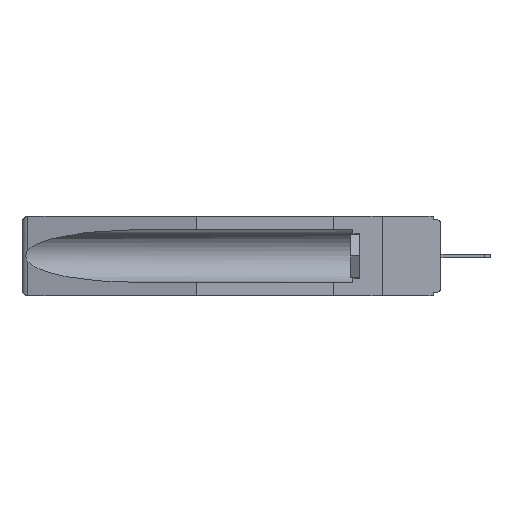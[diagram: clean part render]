
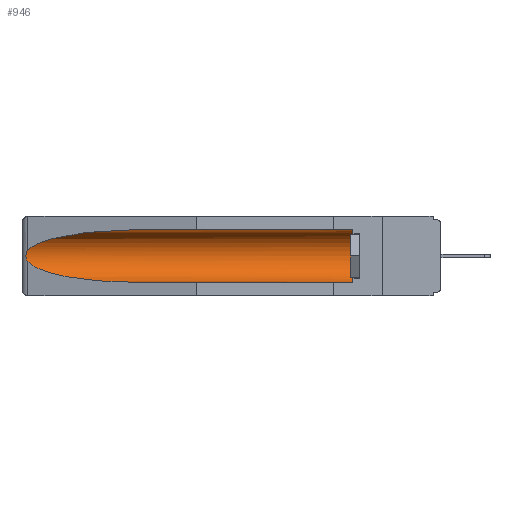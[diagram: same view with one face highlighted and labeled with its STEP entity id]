
A CAD part, left-side view. The second image highlights one B-rep face of the part: STEP entity #946.
In plain terms, the highlighted cylindrical face has radius 2.857 mm (diameter 5.715 mm), a partial arc.
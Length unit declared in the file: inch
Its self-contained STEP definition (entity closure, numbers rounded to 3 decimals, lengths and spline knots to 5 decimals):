
#84 = B_SPLINE_CURVE_WITH_KNOTS ( 'NONE', 3,
 ( #17171, #11885, #2323, #2411, #3823, #6759, #2582, #14613, #9230, #10562 ),
 .UNSPECIFIED., .F., .F.,
 ( 4, 2, 2, 2, 4 ),
 ( 0., 0.00029, 0.00058, 0.00087, 0.00117 ),
 .UNSPECIFIED. ) ;
#172 = VERTEX_POINT ( 'NONE', #4452 ) ;
#292 = CARTESIAN_POINT ( 'NONE',  ( 0.155, 0.126, -0.1715 ) ) ;
#384 = DIRECTION ( 'NONE',  ( 0., -1., 0. ) ) ;
#946 = ADVANCED_FACE ( 'NONE', ( #11473 ), #6060, .F. ) ;
#1336 = CARTESIAN_POINT ( 'NONE',  ( 0.155, -0.30754, -0.284 ) ) ;
#1440 = VECTOR ( 'NONE', #9581, 39.37008 ) ;
#1489 = CARTESIAN_POINT ( 'NONE',  ( 0.155, 1.07973, -0.284 ) ) ;
#1617 = CARTESIAN_POINT ( 'NONE',  ( 0.155, 0.126, -0.284 ) ) ;
#1957 = ORIENTED_EDGE ( 'NONE', *, *, #6160, .F. ) ;
#2323 = CARTESIAN_POINT ( 'NONE',  ( 0.26654, 1.53092, -0.15636 ) ) ;
#2411 = CARTESIAN_POINT ( 'NONE',  ( 0.2673, 1.5327, -0.16383 ) ) ;
#2578 = VECTOR ( 'NONE', #17317, 39.37008 ) ;
#2582 = CARTESIAN_POINT ( 'NONE',  ( 0.2673, 1.53269, -0.17917 ) ) ;
#2665 = ORIENTED_EDGE ( 'NONE', *, *, #8101, .T. ) ;
#2955 = AXIS2_PLACEMENT_3D ( 'NONE', #292, #384, #9781 ) ;
#3110 = CARTESIAN_POINT ( 'NONE',  ( 0.155, 0.126, -0.059 ) ) ;
#3131 = CARTESIAN_POINT ( 'NONE',  ( 0.21114, 1.30732, -0.284 ) ) ;
#3823 = CARTESIAN_POINT ( 'NONE',  ( 0.2675, 1.53308, -0.16763 ) ) ;
#4207 = CARTESIAN_POINT ( 'NONE',  ( 0.155, 1.07973, -0.284 ) ) ;
#4452 = CARTESIAN_POINT ( 'NONE',  ( 0.26537, 1.52718, -0.14972 ) ) ;
#4472 = CARTESIAN_POINT ( 'NONE',  ( 0.26537, 1.52718, -0.19328 ) ) ;
#4498 = ORIENTED_EDGE ( 'NONE', *, *, #11284, .T. ) ;
#4555 = CARTESIAN_POINT ( 'NONE',  ( 0.155, -0.30754, -0.1715 ) ) ;
#5456 = CARTESIAN_POINT ( 'NONE',  ( 0.21114, 1.30732, -0.059 ) ) ;
#5489 = LINE ( 'NONE', #13436, #2578 ) ;
#6060 = CYLINDRICAL_SURFACE ( 'NONE', #16652, 0.1125 ) ;
#6160 = EDGE_CURVE ( 'NONE', #11100, #13497, #9312, .T. ) ;
#6212 = ORIENTED_EDGE ( 'NONE', *, *, #10131, .T. ) ;
#6759 = CARTESIAN_POINT ( 'NONE',  ( 0.2675, 1.53308, -0.17534 ) ) ;
#6836 = VERTEX_POINT ( 'NONE', #14308 ) ;
#8101 = EDGE_CURVE ( 'NONE', #6836, #172, #10718, .T. ) ;
#8758 = CARTESIAN_POINT ( 'NONE',  ( 0.26537, 1.52718, -0.19328 ) ) ;
#9099 = VERTEX_POINT ( 'NONE', #8758 ) ;
#9230 = CARTESIAN_POINT ( 'NONE',  ( 0.26597, 1.5296, -0.19026 ) ) ;
#9312 = LINE ( 'NONE', #1336, #1440 ) ;
#9581 = DIRECTION ( 'NONE',  ( 0., 1., 0. ) ) ;
#9781 = DIRECTION ( 'NONE',  ( 0., 0., 1. ) ) ;
#10131 = EDGE_CURVE ( 'NONE', #11433, #6836, #5489, .T. ) ;
#10562 = CARTESIAN_POINT ( 'NONE',  ( 0.26537, 1.52718, -0.19328 ) ) ;
#10718 =( BOUNDED_CURVE ( )  B_SPLINE_CURVE ( 3, ( #15321, #5456, #12594, #16645 ),
 .UNSPECIFIED., .F., .F. ) 
 B_SPLINE_CURVE_WITH_KNOTS ( ( 4, 4 ),
 ( 4.71239, 6.08839 ),
 .UNSPECIFIED. ) 
 CURVE ( )  GEOMETRIC_REPRESENTATION_ITEM ( )  RATIONAL_B_SPLINE_CURVE ( ( 1., 0.848, 0.848, 1. ) ) 
 REPRESENTATION_ITEM ( '' )  );
#11081 = EDGE_CURVE ( 'NONE', #9099, #13497, #14786, .T. ) ;
#11100 = VERTEX_POINT ( 'NONE', #1617 ) ;
#11284 = EDGE_CURVE ( 'NONE', #172, #9099, #84, .T. ) ;
#11433 = VERTEX_POINT ( 'NONE', #3110 ) ;
#11473 = FACE_OUTER_BOUND ( 'NONE', #13489, .T. ) ;
#11885 = CARTESIAN_POINT ( 'NONE',  ( 0.26597, 1.52961, -0.15275 ) ) ;
#12345 = CARTESIAN_POINT ( 'NONE',  ( 0.25451, 1.48313, -0.24835 ) ) ;
#12435 = DIRECTION ( 'NONE',  ( 0., 0., 1. ) ) ;
#12510 = ORIENTED_EDGE ( 'NONE', *, *, #11081, .T. ) ;
#12594 = CARTESIAN_POINT ( 'NONE',  ( 0.25451, 1.48313, -0.09465 ) ) ;
#12631 = EDGE_CURVE ( 'NONE', #11100, #11433, #17350, .T. ) ;
#12781 = DIRECTION ( 'NONE',  ( 0., 1., 0. ) ) ;
#13436 = CARTESIAN_POINT ( 'NONE',  ( 0.155, -0.30754, -0.059 ) ) ;
#13489 = EDGE_LOOP ( 'NONE', ( #2665, #4498, #12510, #1957, #15232, #6212 ) ) ;
#13497 = VERTEX_POINT ( 'NONE', #1489 ) ;
#14308 = CARTESIAN_POINT ( 'NONE',  ( 0.155, 1.07973, -0.059 ) ) ;
#14613 = CARTESIAN_POINT ( 'NONE',  ( 0.26655, 1.53094, -0.18657 ) ) ;
#14786 =( BOUNDED_CURVE ( )  B_SPLINE_CURVE ( 3, ( #4472, #12345, #3131, #4207 ),
 .UNSPECIFIED., .F., .F. ) 
 B_SPLINE_CURVE_WITH_KNOTS ( ( 4, 4 ),
 ( 0.1948, 1.5708 ),
 .UNSPECIFIED. ) 
 CURVE ( )  GEOMETRIC_REPRESENTATION_ITEM ( )  RATIONAL_B_SPLINE_CURVE ( ( 1., 0.848, 0.848, 1. ) ) 
 REPRESENTATION_ITEM ( '' )  );
#15232 = ORIENTED_EDGE ( 'NONE', *, *, #12631, .T. ) ;
#15321 = CARTESIAN_POINT ( 'NONE',  ( 0.155, 1.07973, -0.059 ) ) ;
#16645 = CARTESIAN_POINT ( 'NONE',  ( 0.26537, 1.52718, -0.14972 ) ) ;
#16652 = AXIS2_PLACEMENT_3D ( 'NONE', #4555, #12781, #12435 ) ;
#17171 = CARTESIAN_POINT ( 'NONE',  ( 0.26537, 1.52718, -0.14972 ) ) ;
#17317 = DIRECTION ( 'NONE',  ( 0., 1., 0. ) ) ;
#17350 = CIRCLE ( 'NONE', #2955, 0.1125 ) ;
